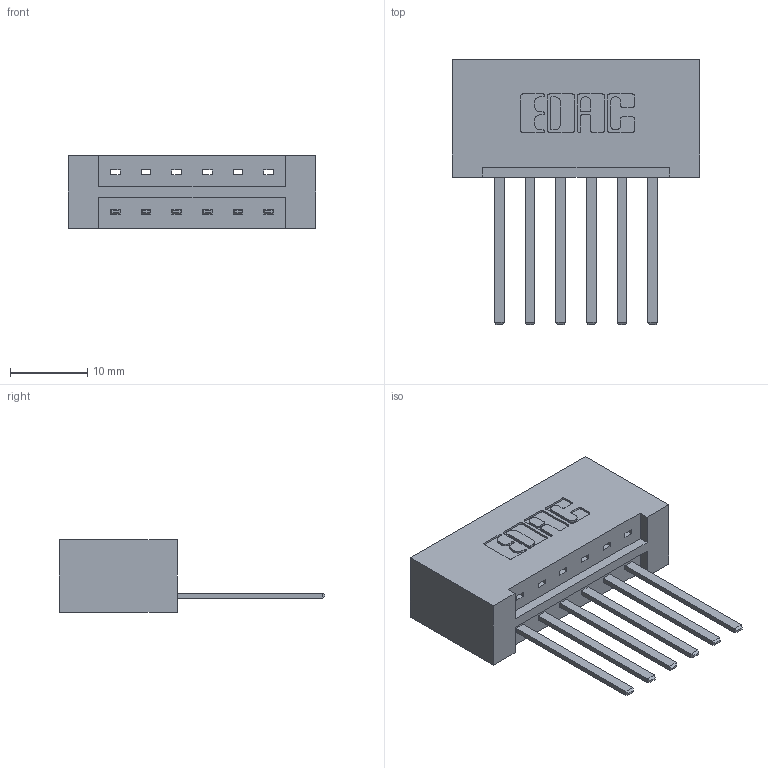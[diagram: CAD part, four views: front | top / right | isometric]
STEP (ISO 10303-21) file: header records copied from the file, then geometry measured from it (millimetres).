
FILE_DESCRIPTION (( 'STEP AP203' ), '1' );
FILE_NAME ('333-006-544-101.STEP', '2018-07-31T21:22:18', ( '' ), ( '' ), 'SwSTEP 2.0', 'SolidWorks 2016', '' );
FILE_SCHEMA (( 'CONFIG_CONTROL_DESIGN' ));
Length unit declared in the file: inch
Products named in the file (3): 345-292-001_345-293-144; 333-006-544-101; 333 Part_Lugless
Assembly tree (7 placements, depth 2):
  333-006-544-101
    333 Part_Lugless
    345-292-001_345-293-144  x6
Bounding box: 32.03 x 34.3 x 9.4 mm (x, y, z)
Volume: 3595.7 mm3; surface area: 3837.3 mm2
Topology: 7 solids, 7 shells, 418 faces, 1235 edges, 814 vertices
Faces by surface type: plane 294, cylinder 124
Entity records: 7863 total; most frequent: CARTESIAN_POINT 1368, ORIENTED_EDGE 1310, DIRECTION 1215, EDGE_CURVE 655, VECTOR 539, LINE 539, VERTEX_POINT 434, AXIS2_PLACEMENT_3D 338
